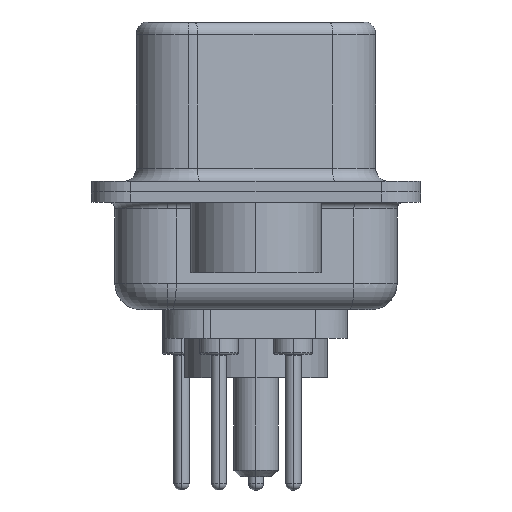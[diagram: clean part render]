
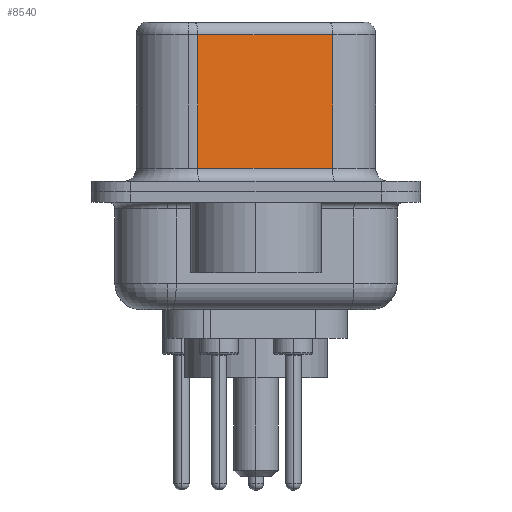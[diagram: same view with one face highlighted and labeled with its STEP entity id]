
A CAD part, left-side view. The second image highlights one B-rep face of the part: STEP entity #8540.
In plain terms, the highlighted planar face has unit normal (-0.985, -0.174, 0).
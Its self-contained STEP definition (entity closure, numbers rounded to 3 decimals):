
#166 = DIRECTION ( 'NONE',  ( 0.174, -0.985, 0. ) ) ;
#3694 = CARTESIAN_POINT ( 'NONE',  ( 3.675, 2.233, 6.52 ) ) ;
#4602 = VERTEX_POINT ( 'NONE', #7315 ) ;
#4717 = EDGE_CURVE ( 'NONE', #11233, #19693, #6814, .T. ) ;
#5823 = DIRECTION ( 'NONE',  ( 0.985, 0.174, 0. ) ) ;
#5987 = VECTOR ( 'NONE', #7704, 1000. ) ;
#6243 = EDGE_LOOP ( 'NONE', ( #18619, #12733, #15812, #6613 ) ) ;
#6613 = ORIENTED_EDGE ( 'NONE', *, *, #18982, .T. ) ;
#6814 = LINE ( 'NONE', #9588, #5987 ) ;
#7315 = CARTESIAN_POINT ( 'NONE',  ( 3.675, 2.233, 6.02 ) ) ;
#7487 = PLANE ( 'NONE',  #9865 ) ;
#7704 = DIRECTION ( 'NONE',  ( 0., 0., -1. ) ) ;
#8540 = ADVANCED_FACE ( 'NONE', ( #22195 ), #7487, .F. ) ;
#9588 = CARTESIAN_POINT ( 'NONE',  ( 4.585, -2.927, 6.52 ) ) ;
#9865 = AXIS2_PLACEMENT_3D ( 'NONE', #10855, #5823, #16614 ) ;
#9999 = DIRECTION ( 'NONE',  ( -0.174, 0.985, 0. ) ) ;
#10855 = CARTESIAN_POINT ( 'NONE',  ( 4.585, -2.927, 6.52 ) ) ;
#11233 = VERTEX_POINT ( 'NONE', #22289 ) ;
#11554 = CARTESIAN_POINT ( 'NONE',  ( 4.585, -2.927, 0.9 ) ) ;
#12371 = VECTOR ( 'NONE', #18142, 1000. ) ;
#12492 = VECTOR ( 'NONE', #166, 1000. ) ;
#12733 = ORIENTED_EDGE ( 'NONE', *, *, #13597, .T. ) ;
#12891 = VERTEX_POINT ( 'NONE', #18056 ) ;
#13534 = EDGE_CURVE ( 'NONE', #4602, #12891, #19705, .T. ) ;
#13597 = EDGE_CURVE ( 'NONE', #11233, #4602, #19099, .T. ) ;
#15543 = LINE ( 'NONE', #18076, #12492 ) ;
#15754 = CARTESIAN_POINT ( 'NONE',  ( 4.585, -2.927, 6.02 ) ) ;
#15812 = ORIENTED_EDGE ( 'NONE', *, *, #13534, .T. ) ;
#16604 = VECTOR ( 'NONE', #9999, 1000. ) ;
#16614 = DIRECTION ( 'NONE',  ( -0.174, 0.985, 0. ) ) ;
#18056 = CARTESIAN_POINT ( 'NONE',  ( 3.675, 2.233, 0.9 ) ) ;
#18076 = CARTESIAN_POINT ( 'NONE',  ( 4.585, -2.927, 0.9 ) ) ;
#18142 = DIRECTION ( 'NONE',  ( 0., 0., -1. ) ) ;
#18619 = ORIENTED_EDGE ( 'NONE', *, *, #4717, .F. ) ;
#18982 = EDGE_CURVE ( 'NONE', #12891, #19693, #15543, .T. ) ;
#19099 = LINE ( 'NONE', #15754, #16604 ) ;
#19693 = VERTEX_POINT ( 'NONE', #11554 ) ;
#19705 = LINE ( 'NONE', #3694, #12371 ) ;
#22195 = FACE_OUTER_BOUND ( 'NONE', #6243, .T. ) ;
#22289 = CARTESIAN_POINT ( 'NONE',  ( 4.585, -2.927, 6.02 ) ) ;
